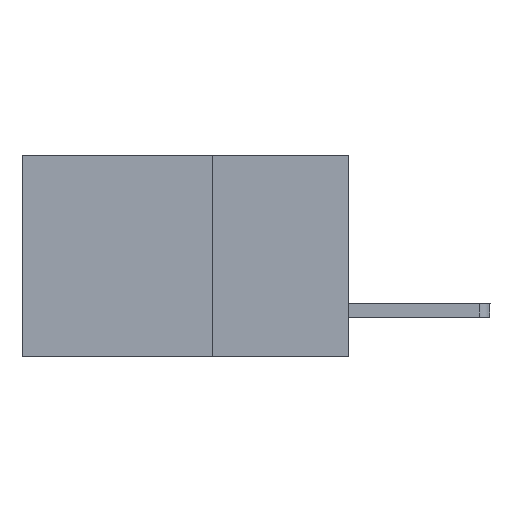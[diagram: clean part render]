
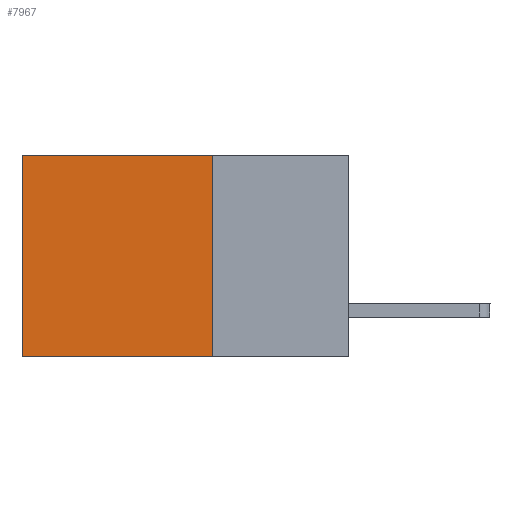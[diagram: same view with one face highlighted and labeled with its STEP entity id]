
A CAD part, left-side view. The second image highlights one B-rep face of the part: STEP entity #7967.
In plain terms, the highlighted planar face has unit normal (-1, 0, 0).
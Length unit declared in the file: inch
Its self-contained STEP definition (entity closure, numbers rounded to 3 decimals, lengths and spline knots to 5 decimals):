
#572 = ORIENTED_EDGE ( 'NONE', *, *, #2713, .F. ) ;
#720 = VECTOR ( 'NONE', #5691, 39.37008 ) ;
#1008 = EDGE_LOOP ( 'NONE', ( #5071, #8763, #572, #4245 ) ) ;
#1377 = EDGE_CURVE ( 'NONE', #6713, #5855, #9039, .T. ) ;
#1509 = CARTESIAN_POINT ( 'NONE',  ( 0.298, 0.25, -0.37 ) ) ;
#2000 = PLANE ( 'NONE',  #5798 ) ;
#2019 = CARTESIAN_POINT ( 'NONE',  ( 0.298, 0.25, 0. ) ) ;
#2030 = EDGE_CURVE ( 'NONE', #4318, #5855, #2100, .T. ) ;
#2100 = LINE ( 'NONE', #2818, #5303 ) ;
#2346 = LINE ( 'NONE', #6624, #720 ) ;
#2686 = DIRECTION ( 'NONE',  ( 0., 1., 0. ) ) ;
#2713 = EDGE_CURVE ( 'NONE', #4334, #6713, #2346, .T. ) ;
#2818 = CARTESIAN_POINT ( 'NONE',  ( 0.298, 0.6, 0. ) ) ;
#3334 = VECTOR ( 'NONE', #2686, 39.37008 ) ;
#4199 = CARTESIAN_POINT ( 'NONE',  ( 0.298, 0.25, 0. ) ) ;
#4245 = ORIENTED_EDGE ( 'NONE', *, *, #8629, .T. ) ;
#4318 = VERTEX_POINT ( 'NONE', #5357 ) ;
#4334 = VERTEX_POINT ( 'NONE', #4199 ) ;
#5071 = ORIENTED_EDGE ( 'NONE', *, *, #2030, .T. ) ;
#5264 = LINE ( 'NONE', #2019, #3334 ) ;
#5303 = VECTOR ( 'NONE', #10393, 39.37008 ) ;
#5352 = DIRECTION ( 'NONE',  ( 1., 0., 0. ) ) ;
#5357 = CARTESIAN_POINT ( 'NONE',  ( 0.298, 0.6, 0. ) ) ;
#5598 = CARTESIAN_POINT ( 'NONE',  ( 0.298, 0.6, -0.37 ) ) ;
#5691 = DIRECTION ( 'NONE',  ( 0., 0., -1. ) ) ;
#5798 = AXIS2_PLACEMENT_3D ( 'NONE', #10460, #5352, #8699 ) ;
#5855 = VERTEX_POINT ( 'NONE', #5598 ) ;
#6624 = CARTESIAN_POINT ( 'NONE',  ( 0.298, 0.25, 0. ) ) ;
#6713 = VERTEX_POINT ( 'NONE', #10818 ) ;
#7748 = VECTOR ( 'NONE', #9916, 39.37008 ) ;
#7967 = ADVANCED_FACE ( 'NONE', ( #10351 ), #2000, .F. ) ;
#8629 = EDGE_CURVE ( 'NONE', #4334, #4318, #5264, .T. ) ;
#8699 = DIRECTION ( 'NONE',  ( 0., 0., -1. ) ) ;
#8763 = ORIENTED_EDGE ( 'NONE', *, *, #1377, .F. ) ;
#9039 = LINE ( 'NONE', #1509, #7748 ) ;
#9916 = DIRECTION ( 'NONE',  ( 0., 1., 0. ) ) ;
#10351 = FACE_OUTER_BOUND ( 'NONE', #1008, .T. ) ;
#10393 = DIRECTION ( 'NONE',  ( 0., 0., -1. ) ) ;
#10460 = CARTESIAN_POINT ( 'NONE',  ( 0.298, 0.25, 0. ) ) ;
#10818 = CARTESIAN_POINT ( 'NONE',  ( 0.298, 0.25, -0.37 ) ) ;
